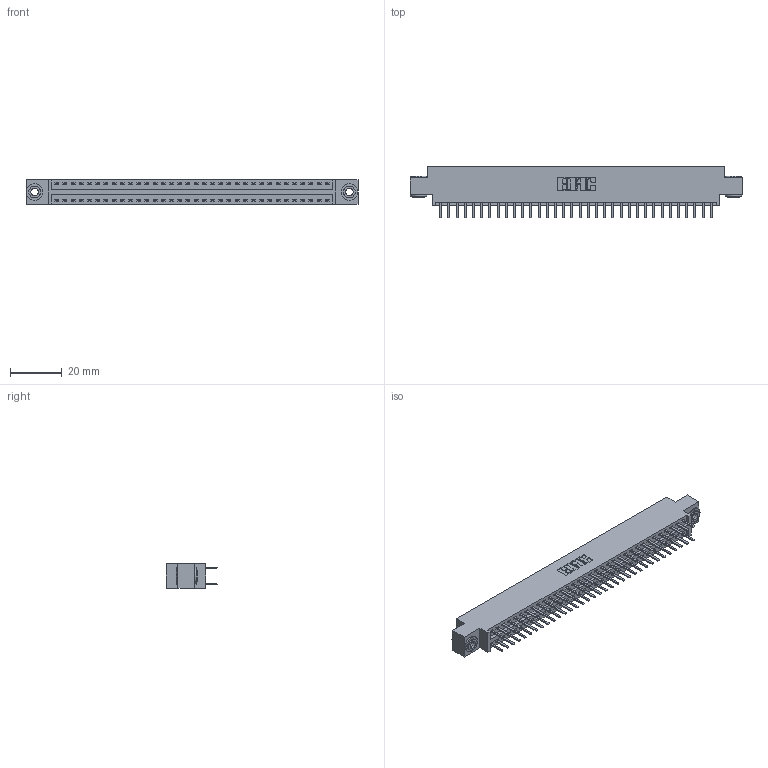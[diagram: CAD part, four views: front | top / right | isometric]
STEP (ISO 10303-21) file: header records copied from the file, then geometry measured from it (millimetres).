
FILE_DESCRIPTION (( 'STEP AP203' ), '1' );
FILE_NAME ('396-068-520-803.STEP', '2019-11-02T10:17:47', ( '' ), ( '' ), 'SwSTEP 2.0', 'SolidWorks 2016', '' );
FILE_SCHEMA (( 'CONFIG_CONTROL_DESIGN' ));
Length unit declared in the file: inch
Products named in the file (4): 346 Part_0.170 Offset - 0.156 Dia-TH; 345-292-001_345-293-120; 345-250-002_345-250-002-102; 396-068-520-803
Assembly tree (71 placements, depth 2):
  396-068-520-803
    346 Part_0.170 Offset - 0.156 Dia-TH
    345-292-001_345-293-120  x68
    345-250-002_345-250-002-102  x2
Bounding box: 128.52 x 20.02 x 9.4 mm (x, y, z)
Volume: 12305.4 mm3; surface area: 17112.7 mm2
Topology: 71 solids, 71 shells, 3972 faces, 11501 edges, 7482 vertices
Faces by surface type: plane 2606, cylinder 1358, cone 8
Entity records: 24162 total; most frequent: CARTESIAN_POINT 3983, ORIENTED_EDGE 3898, DIRECTION 3579, EDGE_CURVE 1949, LINE 1653, VECTOR 1653, VERTEX_POINT 1294, AXIS2_PLACEMENT_3D 963
